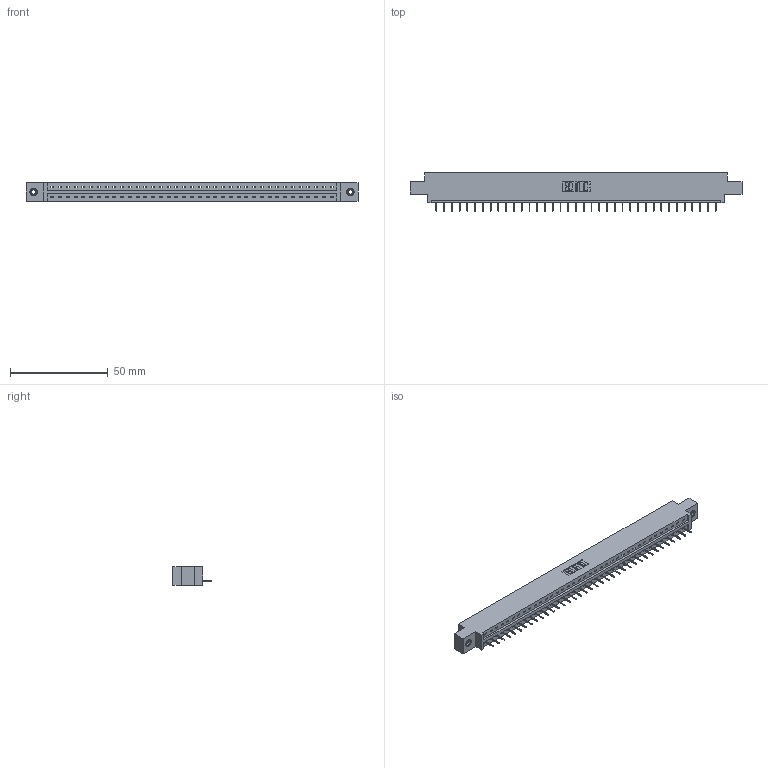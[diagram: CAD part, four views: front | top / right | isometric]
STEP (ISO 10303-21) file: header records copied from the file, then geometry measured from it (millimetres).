
FILE_DESCRIPTION (( 'STEP AP203' ), '1' );
FILE_NAME ('337-037-524-608.STEP', '2019-10-01T15:28:52', ( '' ), ( '' ), 'SwSTEP 2.0', 'SolidWorks 2016', '' );
FILE_SCHEMA (( 'CONFIG_CONTROL_DESIGN' ));
Length unit declared in the file: inch
Products named in the file (4): 345-292-001_345-293-124; 345-250-001_345-250-003-102; 337 Part_0.170 Offset - 0.156 Dia-TI; 337-037-524-608
Assembly tree (40 placements, depth 2):
  337-037-524-608
    337 Part_0.170 Offset - 0.156 Dia-TI
    345-292-001_345-293-124  x37
    345-250-001_345-250-003-102  x2
Bounding box: 169.62 x 19.69 x 9.4 mm (x, y, z)
Volume: 17296.5 mm3; surface area: 17457.8 mm2
Topology: 40 solids, 40 shells, 2620 faces, 7563 edges, 4886 vertices
Faces by surface type: plane 2030, cylinder 574, cone 12, torus 4
Entity records: 29542 total; most frequent: CARTESIAN_POINT 5124, ORIENTED_EDGE 5090, DIRECTION 4357, EDGE_CURVE 2545, LINE 2401, VECTOR 2401, VERTEX_POINT 1688, AXIS2_PLACEMENT_3D 978
